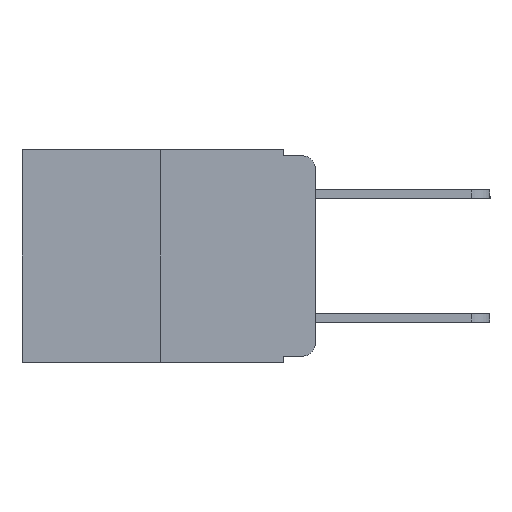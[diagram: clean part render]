
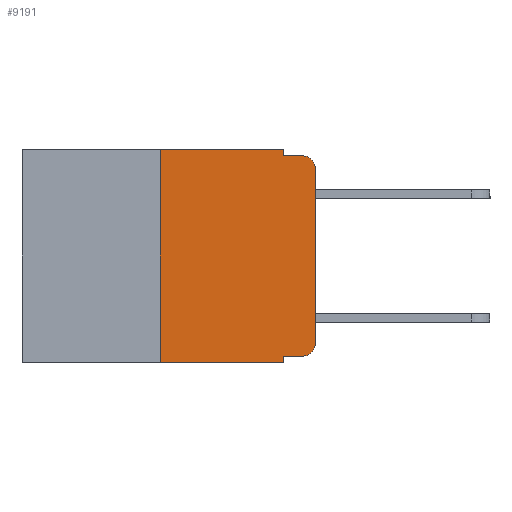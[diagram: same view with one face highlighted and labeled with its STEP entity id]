
A CAD part, left-side view. The second image highlights one B-rep face of the part: STEP entity #9191.
In plain terms, the highlighted planar face has unit normal (-1, 0, 0).
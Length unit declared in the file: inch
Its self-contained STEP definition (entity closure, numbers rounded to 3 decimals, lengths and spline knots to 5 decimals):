
#99 = CARTESIAN_POINT ( 'NONE',  ( 0., 0.25, -0.343 ) ) ;
#176 = ORIENTED_EDGE ( 'NONE', *, *, #8697, .T. ) ;
#312 = DIRECTION ( 'NONE',  ( 0., 0., -1. ) ) ;
#336 = LINE ( 'NONE', #1094, #9244 ) ;
#448 = DIRECTION ( 'NONE',  ( 0., -1., 0. ) ) ;
#697 = CARTESIAN_POINT ( 'NONE',  ( 0., 0.25, 0. ) ) ;
#734 = EDGE_CURVE ( 'NONE', #10536, #9576, #336, .T. ) ;
#763 = AXIS2_PLACEMENT_3D ( 'NONE', #10134, #10042, #10220 ) ;
#765 = CARTESIAN_POINT ( 'NONE',  ( 0., 0.02, -0.333 ) ) ;
#881 = CARTESIAN_POINT ( 'NONE',  ( 0., 0.051, -0.01 ) ) ;
#951 = ORIENTED_EDGE ( 'NONE', *, *, #1660, .F. ) ;
#1075 = DIRECTION ( 'NONE',  ( 0., 0., -1. ) ) ;
#1094 = CARTESIAN_POINT ( 'NONE',  ( 0., 0.051, 0. ) ) ;
#1178 = ORIENTED_EDGE ( 'NONE', *, *, #4756, .T. ) ;
#1222 = VECTOR ( 'NONE', #2672, 39.37008 ) ;
#1372 = ORIENTED_EDGE ( 'NONE', *, *, #734, .F. ) ;
#1401 = VERTEX_POINT ( 'NONE', #3287 ) ;
#1421 = ORIENTED_EDGE ( 'NONE', *, *, #1961, .F. ) ;
#1464 = ORIENTED_EDGE ( 'NONE', *, *, #12048, .T. ) ;
#1660 = EDGE_CURVE ( 'NONE', #10353, #4541, #13323, .T. ) ;
#1961 = EDGE_CURVE ( 'NONE', #4541, #13834, #11647, .T. ) ;
#2481 = EDGE_CURVE ( 'NONE', #13834, #1401, #12745, .T. ) ;
#2672 = DIRECTION ( 'NONE',  ( 0., -1., 0. ) ) ;
#3015 = ORIENTED_EDGE ( 'NONE', *, *, #2481, .F. ) ;
#3209 = EDGE_CURVE ( 'NONE', #1401, #3722, #12338, .T. ) ;
#3287 = CARTESIAN_POINT ( 'NONE',  ( 0., 0.051, -0.01 ) ) ;
#3722 = VERTEX_POINT ( 'NONE', #3930 ) ;
#3930 = CARTESIAN_POINT ( 'NONE',  ( 0., 0.02, -0.01 ) ) ;
#3959 = VECTOR ( 'NONE', #10013, 39.37008 ) ;
#3985 = EDGE_CURVE ( 'NONE', #8271, #3722, #4511, .T. ) ;
#4483 = VECTOR ( 'NONE', #8175, 39.37008 ) ;
#4507 = DIRECTION ( 'NONE',  ( 1., 0., 0. ) ) ;
#4511 = CIRCLE ( 'NONE', #763, 0.02 ) ;
#4541 = VERTEX_POINT ( 'NONE', #6739 ) ;
#4756 = EDGE_CURVE ( 'NONE', #6398, #8271, #6982, .T. ) ;
#5059 = ORIENTED_EDGE ( 'NONE', *, *, #12634, .T. ) ;
#5505 = CARTESIAN_POINT ( 'NONE',  ( 0., 0.051, 0. ) ) ;
#5857 = CARTESIAN_POINT ( 'NONE',  ( 0., 0.473, -0.343 ) ) ;
#6382 = CARTESIAN_POINT ( 'NONE',  ( 0., 0.051, -0.333 ) ) ;
#6398 = VERTEX_POINT ( 'NONE', #12460 ) ;
#6691 = CARTESIAN_POINT ( 'NONE',  ( 0., 0.473, 0. ) ) ;
#6739 = CARTESIAN_POINT ( 'NONE',  ( 0., 0.25, 0. ) ) ;
#6982 = LINE ( 'NONE', #10614, #12063 ) ;
#7408 = LINE ( 'NONE', #9370, #1222 ) ;
#7439 = DIRECTION ( 'NONE',  ( -1., 0., 0. ) ) ;
#7774 = LINE ( 'NONE', #5857, #12642 ) ;
#8125 = CIRCLE ( 'NONE', #10221, 0.02 ) ;
#8175 = DIRECTION ( 'NONE',  ( 0., 0., -1. ) ) ;
#8271 = VERTEX_POINT ( 'NONE', #11579 ) ;
#8320 = DIRECTION ( 'NONE',  ( 0., 0., 1. ) ) ;
#8697 = EDGE_CURVE ( 'NONE', #10353, #9576, #7774, .T. ) ;
#8795 = EDGE_LOOP ( 'NONE', ( #1178, #11178, #9418, #3015, #1421, #951, #176, #1372, #5059, #1464 ) ) ;
#8975 = DIRECTION ( 'NONE',  ( 0., 0., -1. ) ) ;
#9191 = ADVANCED_FACE ( 'NONE', ( #9476 ), #12786, .F. ) ;
#9244 = VECTOR ( 'NONE', #1075, 39.37008 ) ;
#9370 = CARTESIAN_POINT ( 'NONE',  ( 0., 0.051, -0.333 ) ) ;
#9418 = ORIENTED_EDGE ( 'NONE', *, *, #3209, .F. ) ;
#9476 = FACE_OUTER_BOUND ( 'NONE', #8795, .T. ) ;
#9576 = VERTEX_POINT ( 'NONE', #13803 ) ;
#10013 = DIRECTION ( 'NONE',  ( 0., -1., 0. ) ) ;
#10042 = DIRECTION ( 'NONE',  ( -1., 0., 0. ) ) ;
#10134 = CARTESIAN_POINT ( 'NONE',  ( 0., 0.02, -0.03 ) ) ;
#10220 = DIRECTION ( 'NONE',  ( 0., 0., -1. ) ) ;
#10221 = AXIS2_PLACEMENT_3D ( 'NONE', #13271, #7439, #312 ) ;
#10353 = VERTEX_POINT ( 'NONE', #99 ) ;
#10536 = VERTEX_POINT ( 'NONE', #6382 ) ;
#10614 = CARTESIAN_POINT ( 'NONE',  ( 0., 0., 0. ) ) ;
#10953 = VECTOR ( 'NONE', #11495, 39.37008 ) ;
#10999 = CARTESIAN_POINT ( 'NONE',  ( 0., 0.473, 0. ) ) ;
#11178 = ORIENTED_EDGE ( 'NONE', *, *, #3985, .T. ) ;
#11369 = VECTOR ( 'NONE', #448, 39.37008 ) ;
#11377 = AXIS2_PLACEMENT_3D ( 'NONE', #10999, #4507, #8975 ) ;
#11495 = DIRECTION ( 'NONE',  ( 0., 0., 1. ) ) ;
#11579 = CARTESIAN_POINT ( 'NONE',  ( 0., 0., -0.03 ) ) ;
#11647 = LINE ( 'NONE', #6691, #11369 ) ;
#12048 = EDGE_CURVE ( 'NONE', #13846, #6398, #8125, .T. ) ;
#12063 = VECTOR ( 'NONE', #8320, 39.37008 ) ;
#12338 = LINE ( 'NONE', #881, #3959 ) ;
#12460 = CARTESIAN_POINT ( 'NONE',  ( 0., 0., -0.313 ) ) ;
#12634 = EDGE_CURVE ( 'NONE', #10536, #13846, #7408, .T. ) ;
#12642 = VECTOR ( 'NONE', #13815, 39.37008 ) ;
#12745 = LINE ( 'NONE', #13395, #4483 ) ;
#12786 = PLANE ( 'NONE',  #11377 ) ;
#13271 = CARTESIAN_POINT ( 'NONE',  ( 0., 0.02, -0.313 ) ) ;
#13323 = LINE ( 'NONE', #697, #10953 ) ;
#13395 = CARTESIAN_POINT ( 'NONE',  ( 0., 0.051, 0. ) ) ;
#13803 = CARTESIAN_POINT ( 'NONE',  ( 0., 0.051, -0.343 ) ) ;
#13815 = DIRECTION ( 'NONE',  ( 0., -1., 0. ) ) ;
#13834 = VERTEX_POINT ( 'NONE', #5505 ) ;
#13846 = VERTEX_POINT ( 'NONE', #765 ) ;
